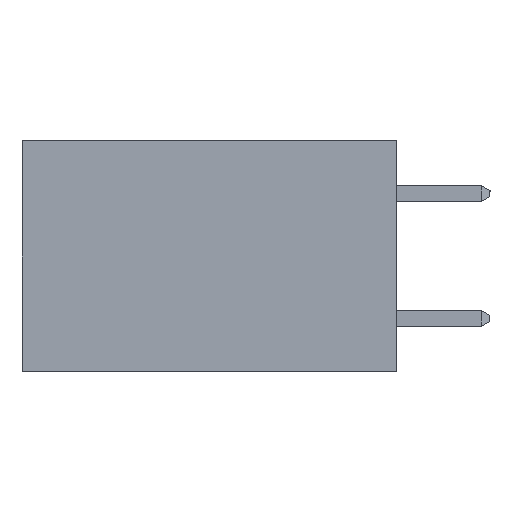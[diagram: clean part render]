
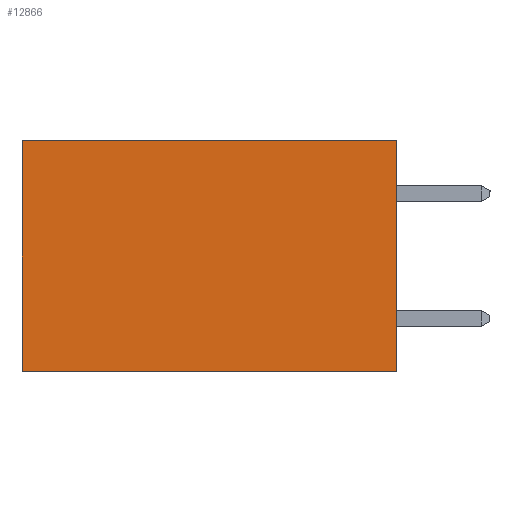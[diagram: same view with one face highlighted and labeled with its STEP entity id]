
A CAD part, left-side view. The second image highlights one B-rep face of the part: STEP entity #12866.
In plain terms, the highlighted planar face has unit normal (-1, 0, 0).
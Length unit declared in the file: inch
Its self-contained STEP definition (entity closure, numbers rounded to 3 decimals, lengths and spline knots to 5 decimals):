
#615 = CARTESIAN_POINT ( 'NONE',  ( 0.2615, 0., -0.37 ) ) ;
#1009 = CARTESIAN_POINT ( 'NONE',  ( 0.2615, 0.6, 0. ) ) ;
#2701 = ORIENTED_EDGE ( 'NONE', *, *, #6068, .F. ) ;
#2838 = DIRECTION ( 'NONE',  ( 0., 0., -1. ) ) ;
#2929 = VECTOR ( 'NONE', #2838, 39.37008 ) ;
#5269 = VECTOR ( 'NONE', #16185, 39.37008 ) ;
#5800 = EDGE_CURVE ( 'NONE', #20844, #20085, #17857, .T. ) ;
#6068 = EDGE_CURVE ( 'NONE', #9296, #20844, #19129, .T. ) ;
#6201 = DIRECTION ( 'NONE',  ( 0., 1., 0. ) ) ;
#7057 = PLANE ( 'NONE',  #24549 ) ;
#7293 = VERTEX_POINT ( 'NONE', #1009 ) ;
#7337 = LINE ( 'NONE', #15084, #2929 ) ;
#8564 = DIRECTION ( 'NONE',  ( 1., 0., 0. ) ) ;
#9296 = VERTEX_POINT ( 'NONE', #12984 ) ;
#9303 = DIRECTION ( 'NONE',  ( 0., 0., -1. ) ) ;
#9314 = CARTESIAN_POINT ( 'NONE',  ( 0.2615, 0., -0.37 ) ) ;
#10274 = CARTESIAN_POINT ( 'NONE',  ( 0.2615, 0., 0. ) ) ;
#11022 = ORIENTED_EDGE ( 'NONE', *, *, #14921, .T. ) ;
#12866 = ADVANCED_FACE ( 'NONE', ( #14295 ), #7057, .F. ) ;
#12984 = CARTESIAN_POINT ( 'NONE',  ( 0.2615, 0., 0. ) ) ;
#13415 = VECTOR ( 'NONE', #9303, 39.37008 ) ;
#14295 = FACE_OUTER_BOUND ( 'NONE', #21914, .T. ) ;
#14921 = EDGE_CURVE ( 'NONE', #7293, #20085, #7337, .T. ) ;
#15084 = CARTESIAN_POINT ( 'NONE',  ( 0.2615, 0.6, -0.37 ) ) ;
#15237 = ORIENTED_EDGE ( 'NONE', *, *, #18789, .T. ) ;
#15288 = VECTOR ( 'NONE', #6201, 39.37008 ) ;
#15892 = LINE ( 'NONE', #10274, #15288 ) ;
#16185 = DIRECTION ( 'NONE',  ( 0., 1., 0. ) ) ;
#16466 = CARTESIAN_POINT ( 'NONE',  ( 0.2615, 0., -0.37 ) ) ;
#16728 = DIRECTION ( 'NONE',  ( 0., 0., -1. ) ) ;
#17857 = LINE ( 'NONE', #615, #5269 ) ;
#18789 = EDGE_CURVE ( 'NONE', #9296, #7293, #15892, .T. ) ;
#19129 = LINE ( 'NONE', #23251, #13415 ) ;
#20085 = VERTEX_POINT ( 'NONE', #22975 ) ;
#20840 = ORIENTED_EDGE ( 'NONE', *, *, #5800, .F. ) ;
#20844 = VERTEX_POINT ( 'NONE', #9314 ) ;
#21914 = EDGE_LOOP ( 'NONE', ( #11022, #20840, #2701, #15237 ) ) ;
#22975 = CARTESIAN_POINT ( 'NONE',  ( 0.2615, 0.6, -0.37 ) ) ;
#23251 = CARTESIAN_POINT ( 'NONE',  ( 0.2615, 0., -0.37 ) ) ;
#24549 = AXIS2_PLACEMENT_3D ( 'NONE', #16466, #8564, #16728 ) ;
